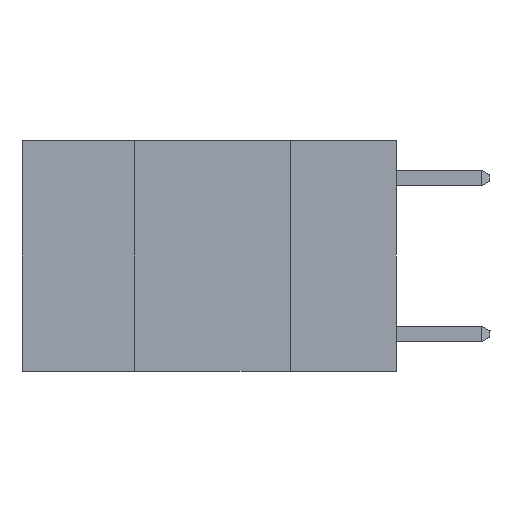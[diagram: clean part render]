
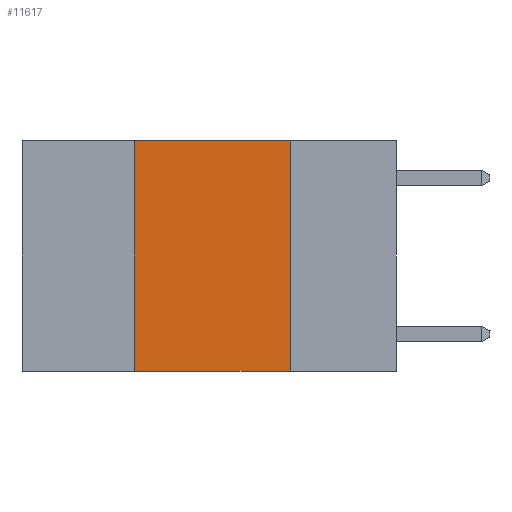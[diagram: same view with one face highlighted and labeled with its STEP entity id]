
A CAD part, left-side view. The second image highlights one B-rep face of the part: STEP entity #11617.
In plain terms, the highlighted planar face has unit normal (-1, 0, 0).
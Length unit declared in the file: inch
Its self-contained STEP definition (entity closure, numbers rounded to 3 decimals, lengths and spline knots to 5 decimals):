
#305 = VERTEX_POINT ( 'NONE', #9614 ) ;
#339 = VECTOR ( 'NONE', #1744, 39.37008 ) ;
#971 = EDGE_LOOP ( 'NONE', ( #8702, #1906, #22104, #7379 ) ) ;
#1449 = EDGE_CURVE ( 'NONE', #27095, #305, #12517, .T. ) ;
#1744 = DIRECTION ( 'NONE',  ( 0., 0., -1. ) ) ;
#1906 = ORIENTED_EDGE ( 'NONE', *, *, #22484, .F. ) ;
#3198 = DIRECTION ( 'NONE',  ( 0., -1., 0. ) ) ;
#3480 = CARTESIAN_POINT ( 'NONE',  ( 0., 0.42, -0.37 ) ) ;
#4473 = DIRECTION ( 'NONE',  ( 0., 0., 1. ) ) ;
#7379 = ORIENTED_EDGE ( 'NONE', *, *, #11628, .T. ) ;
#8272 = VECTOR ( 'NONE', #4473, 39.37008 ) ;
#8702 = ORIENTED_EDGE ( 'NONE', *, *, #1449, .F. ) ;
#9614 = CARTESIAN_POINT ( 'NONE',  ( 0., 0.17, -0.37 ) ) ;
#11461 = CARTESIAN_POINT ( 'NONE',  ( 0., 0.6, -0.37 ) ) ;
#11617 = ADVANCED_FACE ( 'NONE', ( #23501 ), #20330, .F. ) ;
#11628 = EDGE_CURVE ( 'NONE', #17896, #305, #18981, .T. ) ;
#12517 = LINE ( 'NONE', #26474, #339 ) ;
#13651 = DIRECTION ( 'NONE',  ( 1., 0., 0. ) ) ;
#14605 = CARTESIAN_POINT ( 'NONE',  ( 0., 0.6, 0. ) ) ;
#15410 = EDGE_CURVE ( 'NONE', #17896, #20395, #24348, .T. ) ;
#15864 = CARTESIAN_POINT ( 'NONE',  ( 0., 0.42, 0. ) ) ;
#17896 = VERTEX_POINT ( 'NONE', #3480 ) ;
#18656 = LINE ( 'NONE', #14605, #23845 ) ;
#18981 = LINE ( 'NONE', #11461, #22107 ) ;
#20330 = PLANE ( 'NONE',  #27542 ) ;
#20395 = VERTEX_POINT ( 'NONE', #20648 ) ;
#20648 = CARTESIAN_POINT ( 'NONE',  ( 0., 0.42, 0. ) ) ;
#22104 = ORIENTED_EDGE ( 'NONE', *, *, #15410, .F. ) ;
#22107 = VECTOR ( 'NONE', #24865, 39.37008 ) ;
#22269 = CARTESIAN_POINT ( 'NONE',  ( 0., 0.17, 0. ) ) ;
#22484 = EDGE_CURVE ( 'NONE', #20395, #27095, #18656, .T. ) ;
#23501 = FACE_OUTER_BOUND ( 'NONE', #971, .T. ) ;
#23845 = VECTOR ( 'NONE', #3198, 39.37008 ) ;
#24348 = LINE ( 'NONE', #15864, #8272 ) ;
#24769 = CARTESIAN_POINT ( 'NONE',  ( 0., 0.6, 0. ) ) ;
#24865 = DIRECTION ( 'NONE',  ( 0., -1., 0. ) ) ;
#26474 = CARTESIAN_POINT ( 'NONE',  ( 0., 0.17, 0. ) ) ;
#27095 = VERTEX_POINT ( 'NONE', #22269 ) ;
#27319 = DIRECTION ( 'NONE',  ( 0., 0., -1. ) ) ;
#27542 = AXIS2_PLACEMENT_3D ( 'NONE', #24769, #13651, #27319 ) ;
